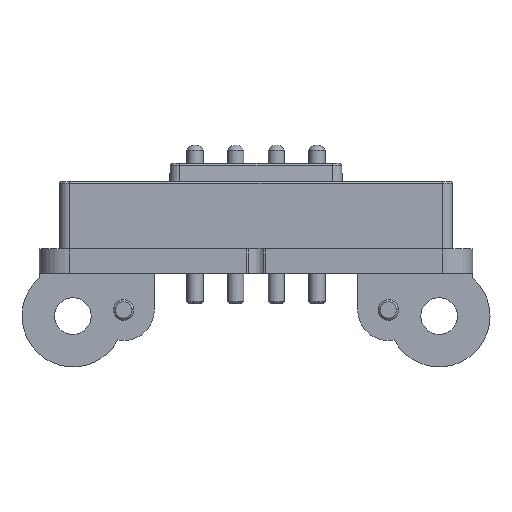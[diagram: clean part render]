
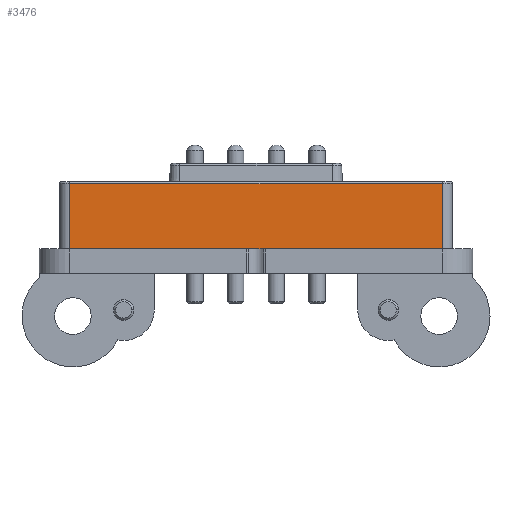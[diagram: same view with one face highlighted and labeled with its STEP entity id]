
A CAD part, front view. The second image highlights one B-rep face of the part: STEP entity #3476.
In plain terms, the highlighted planar face has unit normal (0, -1, 0).
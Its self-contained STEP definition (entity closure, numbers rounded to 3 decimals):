
#295 = DIRECTION ( 'NONE',  ( 0., 0., 1. ) ) ;
#382 = VECTOR ( 'NONE', #295, 1000. ) ;
#640 = CARTESIAN_POINT ( 'NONE',  ( -9.15, -2.05, -0.1 ) ) ;
#912 = FACE_OUTER_BOUND ( 'NONE', #1467, .T. ) ;
#991 = CARTESIAN_POINT ( 'NONE',  ( -9.15, -2.05, -3.3 ) ) ;
#1216 = VECTOR ( 'NONE', #6474, 1000. ) ;
#1467 = EDGE_LOOP ( 'NONE', ( #9082, #5603, #4673, #2956 ) ) ;
#1778 = VERTEX_POINT ( 'NONE', #8549 ) ;
#2544 = DIRECTION ( 'NONE',  ( 1., 0., 0. ) ) ;
#2597 = LINE ( 'NONE', #991, #7402 ) ;
#2941 = LINE ( 'NONE', #5629, #1216 ) ;
#2956 = ORIENTED_EDGE ( 'NONE', *, *, #6808, .T. ) ;
#3401 = EDGE_CURVE ( 'NONE', #1778, #7386, #4482, .T. ) ;
#3476 = ADVANCED_FACE ( 'NONE', ( #912 ), #7048, .F. ) ;
#4152 = EDGE_CURVE ( 'NONE', #7080, #1778, #2597, .T. ) ;
#4354 = EDGE_CURVE ( 'NONE', #7476, #7080, #4945, .T. ) ;
#4482 = LINE ( 'NONE', #5309, #382 ) ;
#4673 = ORIENTED_EDGE ( 'NONE', *, *, #3401, .T. ) ;
#4945 = LINE ( 'NONE', #640, #6156 ) ;
#5309 = CARTESIAN_POINT ( 'NONE',  ( 9.15, -2.05, -3.3 ) ) ;
#5394 = CARTESIAN_POINT ( 'NONE',  ( 9.15, -2.05, -0.1 ) ) ;
#5603 = ORIENTED_EDGE ( 'NONE', *, *, #4152, .T. ) ;
#5629 = CARTESIAN_POINT ( 'NONE',  ( 9.15, -2.05, -0.1 ) ) ;
#6084 = CARTESIAN_POINT ( 'NONE',  ( -9.15, -2.05, -3.3 ) ) ;
#6156 = VECTOR ( 'NONE', #10809, 1000. ) ;
#6262 = AXIS2_PLACEMENT_3D ( 'NONE', #7937, #10509, #10451 ) ;
#6474 = DIRECTION ( 'NONE',  ( -1., 0., 0. ) ) ;
#6808 = EDGE_CURVE ( 'NONE', #7386, #7476, #2941, .T. ) ;
#7048 = PLANE ( 'NONE',  #6262 ) ;
#7080 = VERTEX_POINT ( 'NONE', #6084 ) ;
#7386 = VERTEX_POINT ( 'NONE', #5394 ) ;
#7402 = VECTOR ( 'NONE', #2544, 1000. ) ;
#7476 = VERTEX_POINT ( 'NONE', #9347 ) ;
#7937 = CARTESIAN_POINT ( 'NONE',  ( 0., -2.05, -1.7 ) ) ;
#8549 = CARTESIAN_POINT ( 'NONE',  ( 9.15, -2.05, -3.3 ) ) ;
#9082 = ORIENTED_EDGE ( 'NONE', *, *, #4354, .T. ) ;
#9347 = CARTESIAN_POINT ( 'NONE',  ( -9.15, -2.05, -0.1 ) ) ;
#10451 = DIRECTION ( 'NONE',  ( 1., 0., 0. ) ) ;
#10509 = DIRECTION ( 'NONE',  ( 0., 1., 0. ) ) ;
#10809 = DIRECTION ( 'NONE',  ( 0., 0., -1. ) ) ;
